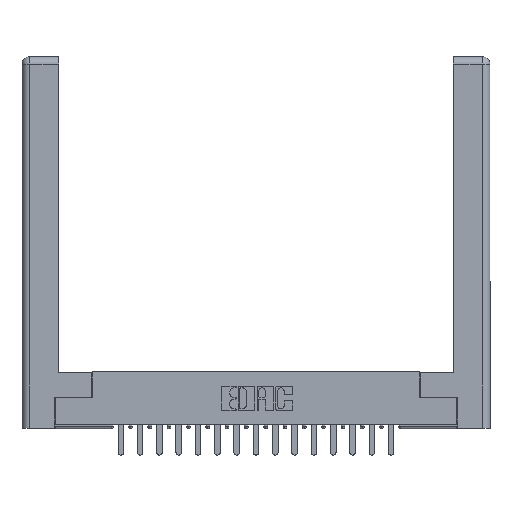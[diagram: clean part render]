
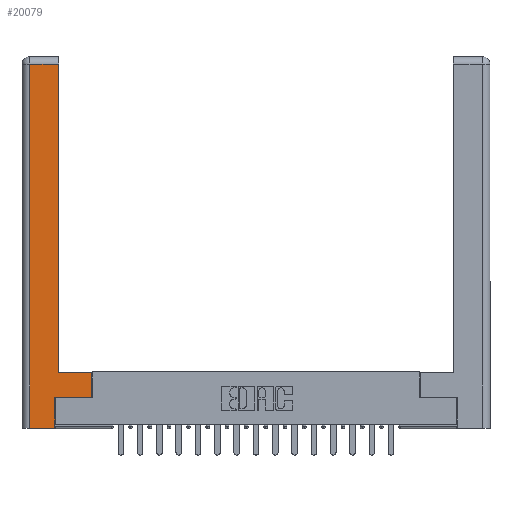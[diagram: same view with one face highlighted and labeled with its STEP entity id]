
A CAD part, top view. The second image highlights one B-rep face of the part: STEP entity #20079.
In plain terms, the highlighted planar face has unit normal (0, 0, 1).
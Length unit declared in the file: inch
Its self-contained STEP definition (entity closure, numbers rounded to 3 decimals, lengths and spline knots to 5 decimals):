
#579 = ORIENTED_EDGE ( 'NONE', *, *, #21533, .T. ) ;
#2200 = EDGE_LOOP ( 'NONE', ( #3014, #20071, #7501, #10206, #579, #16283, #18801, #6707 ) ) ;
#2347 = DIRECTION ( 'NONE',  ( -1., 0., 0. ) ) ;
#2813 = LINE ( 'NONE', #18460, #5761 ) ;
#3014 = ORIENTED_EDGE ( 'NONE', *, *, #14341, .T. ) ;
#3123 = CARTESIAN_POINT ( 'NONE',  ( 0.295, 3., 0. ) ) ;
#3212 = VERTEX_POINT ( 'NONE', #21074 ) ;
#3574 = VECTOR ( 'NONE', #5117, 39.37008 ) ;
#3983 = LINE ( 'NONE', #9094, #15435 ) ;
#4180 = FACE_OUTER_BOUND ( 'NONE', #2200, .T. ) ;
#4996 = EDGE_CURVE ( 'NONE', #18490, #6097, #3983, .T. ) ;
#5117 = DIRECTION ( 'NONE',  ( 0., 1., 0. ) ) ;
#5352 = DIRECTION ( 'NONE',  ( 0., -1., 0. ) ) ;
#5697 = VERTEX_POINT ( 'NONE', #20492 ) ;
#5700 = CARTESIAN_POINT ( 'NONE',  ( 0.0615, 2.94, 0. ) ) ;
#5761 = VECTOR ( 'NONE', #18223, 39.37008 ) ;
#6097 = VERTEX_POINT ( 'NONE', #8977 ) ;
#6202 = LINE ( 'NONE', #3123, #11817 ) ;
#6237 = LINE ( 'NONE', #12820, #14241 ) ;
#6588 = EDGE_CURVE ( 'NONE', #5697, #18490, #10995, .T. ) ;
#6707 = ORIENTED_EDGE ( 'NONE', *, *, #12715, .T. ) ;
#7501 = ORIENTED_EDGE ( 'NONE', *, *, #8109, .T. ) ;
#8105 = LINE ( 'NONE', #20320, #3574 ) ;
#8109 = EDGE_CURVE ( 'NONE', #8486, #19698, #15547, .T. ) ;
#8173 = LINE ( 'NONE', #5700, #9480 ) ;
#8178 = DIRECTION ( 'NONE',  ( -1., 0., 0. ) ) ;
#8486 = VERTEX_POINT ( 'NONE', #18449 ) ;
#8977 = CARTESIAN_POINT ( 'NONE',  ( 0.565, 0.45, 0. ) ) ;
#8989 = CARTESIAN_POINT ( 'NONE',  ( 0.0615, 0., 0. ) ) ;
#9094 = CARTESIAN_POINT ( 'NONE',  ( 0.565, 0.45, 0. ) ) ;
#9167 = DIRECTION ( 'NONE',  ( 1., 0., 0. ) ) ;
#9480 = VECTOR ( 'NONE', #2347, 39.37008 ) ;
#9673 = CARTESIAN_POINT ( 'NONE',  ( 0.565, 0.245, 0. ) ) ;
#9968 = DIRECTION ( 'NONE',  ( 0., 1., 0. ) ) ;
#10206 = ORIENTED_EDGE ( 'NONE', *, *, #13373, .T. ) ;
#10632 = DIRECTION ( 'NONE',  ( 0., 1., 0. ) ) ;
#10995 = LINE ( 'NONE', #17110, #21382 ) ;
#11762 = EDGE_CURVE ( 'NONE', #15166, #8486, #8173, .T. ) ;
#11817 = VECTOR ( 'NONE', #9968, 39.37008 ) ;
#12715 = EDGE_CURVE ( 'NONE', #6097, #16773, #2813, .T. ) ;
#12820 = CARTESIAN_POINT ( 'NONE',  ( 0.265, 0., 0. ) ) ;
#13373 = EDGE_CURVE ( 'NONE', #19698, #3212, #6237, .T. ) ;
#14083 = DIRECTION ( 'NONE',  ( 1., 0., 0. ) ) ;
#14241 = VECTOR ( 'NONE', #9167, 39.37008 ) ;
#14341 = EDGE_CURVE ( 'NONE', #16773, #15166, #6202, .T. ) ;
#15166 = VERTEX_POINT ( 'NONE', #16236 ) ;
#15435 = VECTOR ( 'NONE', #10632, 39.37008 ) ;
#15547 = LINE ( 'NONE', #8989, #19294 ) ;
#15619 = CARTESIAN_POINT ( 'NONE',  ( 0.0615, 0., 0. ) ) ;
#16236 = CARTESIAN_POINT ( 'NONE',  ( 0.295, 2.94, 0. ) ) ;
#16283 = ORIENTED_EDGE ( 'NONE', *, *, #6588, .T. ) ;
#16773 = VERTEX_POINT ( 'NONE', #20799 ) ;
#16781 = PLANE ( 'NONE',  #18034 ) ;
#17110 = CARTESIAN_POINT ( 'NONE',  ( 0.565, 0.245, 0. ) ) ;
#18034 = AXIS2_PLACEMENT_3D ( 'NONE', #18607, #21717, #8178 ) ;
#18223 = DIRECTION ( 'NONE',  ( -1., 0., 0. ) ) ;
#18449 = CARTESIAN_POINT ( 'NONE',  ( 0.0615, 2.94, 0. ) ) ;
#18460 = CARTESIAN_POINT ( 'NONE',  ( 0.295, 0.45, 0. ) ) ;
#18490 = VERTEX_POINT ( 'NONE', #9673 ) ;
#18607 = CARTESIAN_POINT ( 'NONE',  ( 0., 0., 0. ) ) ;
#18801 = ORIENTED_EDGE ( 'NONE', *, *, #4996, .T. ) ;
#19294 = VECTOR ( 'NONE', #5352, 39.37008 ) ;
#19698 = VERTEX_POINT ( 'NONE', #15619 ) ;
#20071 = ORIENTED_EDGE ( 'NONE', *, *, #11762, .T. ) ;
#20079 = ADVANCED_FACE ( 'NONE', ( #4180 ), #16781, .F. ) ;
#20320 = CARTESIAN_POINT ( 'NONE',  ( 0.265, 0.245, 0. ) ) ;
#20492 = CARTESIAN_POINT ( 'NONE',  ( 0.265, 0.245, 0. ) ) ;
#20799 = CARTESIAN_POINT ( 'NONE',  ( 0.295, 0.45, 0. ) ) ;
#21074 = CARTESIAN_POINT ( 'NONE',  ( 0.265, 0., 0. ) ) ;
#21382 = VECTOR ( 'NONE', #14083, 39.37008 ) ;
#21533 = EDGE_CURVE ( 'NONE', #3212, #5697, #8105, .T. ) ;
#21717 = DIRECTION ( 'NONE',  ( 0., 0., -1. ) ) ;
